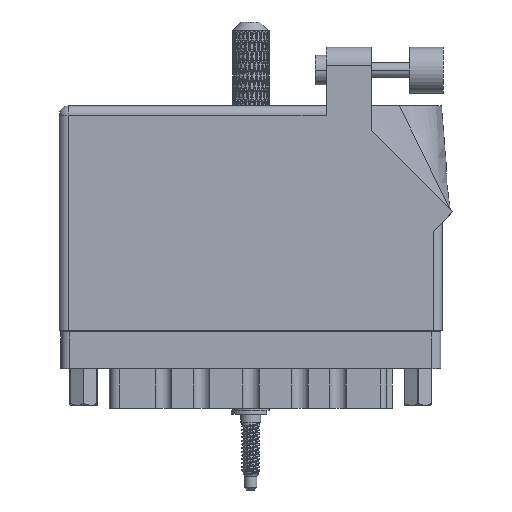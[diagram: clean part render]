
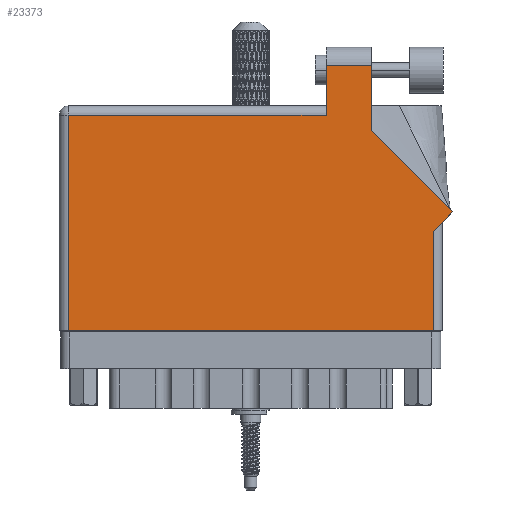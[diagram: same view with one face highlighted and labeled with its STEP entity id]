
A CAD part, front view. The second image highlights one B-rep face of the part: STEP entity #23373.
In plain terms, the highlighted face is planar.
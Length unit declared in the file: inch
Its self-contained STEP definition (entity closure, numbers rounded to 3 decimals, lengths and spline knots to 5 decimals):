
#1160 = DIRECTION ( 'NONE',  ( 0., 0., -1. ) ) ;
#1445 = VERTEX_POINT ( 'NONE', #15728 ) ;
#2718 = CARTESIAN_POINT ( 'NONE',  ( 0.062, 0., 0. ) ) ;
#2809 = CARTESIAN_POINT ( 'NONE',  ( 2.55, 0., 0. ) ) ;
#8725 = EDGE_CURVE ( 'NONE', #46012, #100111, #115693, .T. ) ;
#9694 = DIRECTION ( 'NONE',  ( 1., 0., 0. ) ) ;
#10680 = DIRECTION ( 'NONE',  ( -1., 0., 0. ) ) ;
#15728 = CARTESIAN_POINT ( 'NONE',  ( 2.55, 0.675, 0. ) ) ;
#22174 = LINE ( 'NONE', #75197, #93728 ) ;
#22695 = DIRECTION ( 'NONE',  ( 0., 1., 0. ) ) ;
#23373 = ADVANCED_FACE ( 'NONE', ( #100048 ), #78764, .F. ) ;
#23724 = VECTOR ( 'NONE', #22695, 39.37008 ) ;
#24155 = EDGE_CURVE ( 'NONE', #119926, #46796, #34147, .T. ) ;
#25047 = LINE ( 'NONE', #74549, #72838 ) ;
#26389 = LINE ( 'NONE', #67355, #39876 ) ;
#30416 = CARTESIAN_POINT ( 'NONE',  ( 0., 1.468, 0. ) ) ;
#32674 = CARTESIAN_POINT ( 'NONE',  ( 2.68271, 0.80771, 0. ) ) ;
#34147 = LINE ( 'NONE', #80301, #23724 ) ;
#36183 = DIRECTION ( 'NONE',  ( 0.707, 0.707, 0. ) ) ;
#39404 = CARTESIAN_POINT ( 'NONE',  ( 0., 0., 0. ) ) ;
#39876 = VECTOR ( 'NONE', #46555, 39.37008 ) ;
#40272 = DIRECTION ( 'NONE',  ( -0.707, 0.707, 0. ) ) ;
#43298 = ORIENTED_EDGE ( 'NONE', *, *, #79503, .T. ) ;
#46012 = VERTEX_POINT ( 'NONE', #2718 ) ;
#46555 = DIRECTION ( 'NONE',  ( 0., -1., 0. ) ) ;
#46796 = VERTEX_POINT ( 'NONE', #100819 ) ;
#49340 = EDGE_CURVE ( 'NONE', #68187, #119926, #106894, .T. ) ;
#50073 = ORIENTED_EDGE ( 'NONE', *, *, #8725, .T. ) ;
#50789 = CARTESIAN_POINT ( 'NONE',  ( 0., 1.53, 0. ) ) ;
#54359 = VERTEX_POINT ( 'NONE', #75942 ) ;
#60581 = CARTESIAN_POINT ( 'NONE',  ( 2.55, 0.737, 0. ) ) ;
#61415 = VECTOR ( 'NONE', #120790, 39.37008 ) ;
#67150 = DIRECTION ( 'NONE',  ( -1., 0., 0. ) ) ;
#67355 = CARTESIAN_POINT ( 'NONE',  ( 0.062, 0., 0. ) ) ;
#68187 = VERTEX_POINT ( 'NONE', #120037 ) ;
#69069 = EDGE_CURVE ( 'NONE', #54359, #46012, #26389, .T. ) ;
#70728 = ORIENTED_EDGE ( 'NONE', *, *, #115049, .T. ) ;
#72074 = CARTESIAN_POINT ( 'NONE',  ( 1.819, 1.805, 0. ) ) ;
#72685 = CARTESIAN_POINT ( 'NONE',  ( 1.819, 1.468, 0. ) ) ;
#72838 = VECTOR ( 'NONE', #36183, 39.37008 ) ;
#74119 = EDGE_CURVE ( 'NONE', #46796, #106268, #95720, .T. ) ;
#74367 = ORIENTED_EDGE ( 'NONE', *, *, #49340, .T. ) ;
#74549 = CARTESIAN_POINT ( 'NONE',  ( 2.612, 0.737, 0. ) ) ;
#75197 = CARTESIAN_POINT ( 'NONE',  ( 1.819, 1.53, 0. ) ) ;
#75942 = CARTESIAN_POINT ( 'NONE',  ( 0.062, 1.468, 0. ) ) ;
#76597 = ORIENTED_EDGE ( 'NONE', *, *, #69069, .T. ) ;
#78764 = PLANE ( 'NONE',  #100450 ) ;
#79074 = ORIENTED_EDGE ( 'NONE', *, *, #114481, .T. ) ;
#79503 = EDGE_CURVE ( 'NONE', #100111, #1445, #104712, .T. ) ;
#80206 = DIRECTION ( 'NONE',  ( 0., 1., 0. ) ) ;
#80301 = CARTESIAN_POINT ( 'NONE',  ( 2.126, 1.36442, 0. ) ) ;
#83221 = VECTOR ( 'NONE', #67150, 39.37008 ) ;
#90413 = VECTOR ( 'NONE', #9694, 39.37008 ) ;
#90846 = EDGE_CURVE ( 'NONE', #111351, #54359, #118954, .T. ) ;
#91414 = VECTOR ( 'NONE', #80206, 39.37008 ) ;
#93728 = VECTOR ( 'NONE', #105547, 39.37008 ) ;
#95720 = LINE ( 'NONE', #72074, #61415 ) ;
#100048 = FACE_OUTER_BOUND ( 'NONE', #108506, .T. ) ;
#100111 = VERTEX_POINT ( 'NONE', #2809 ) ;
#100450 = AXIS2_PLACEMENT_3D ( 'NONE', #50789, #1160, #10680 ) ;
#100819 = CARTESIAN_POINT ( 'NONE',  ( 2.126, 1.805, 0. ) ) ;
#104712 = LINE ( 'NONE', #60581, #91414 ) ;
#105547 = DIRECTION ( 'NONE',  ( 0., -1., 0. ) ) ;
#106268 = VERTEX_POINT ( 'NONE', #114165 ) ;
#106894 = LINE ( 'NONE', #32674, #111502 ) ;
#107000 = ORIENTED_EDGE ( 'NONE', *, *, #90846, .T. ) ;
#108506 = EDGE_LOOP ( 'NONE', ( #117914, #122545, #79074, #107000, #76597, #50073, #43298, #70728, #74367 ) ) ;
#110491 = CARTESIAN_POINT ( 'NONE',  ( 2.126, 1.36442, 0. ) ) ;
#111351 = VERTEX_POINT ( 'NONE', #72685 ) ;
#111502 = VECTOR ( 'NONE', #40272, 39.37008 ) ;
#114165 = CARTESIAN_POINT ( 'NONE',  ( 1.819, 1.805, 0. ) ) ;
#114481 = EDGE_CURVE ( 'NONE', #106268, #111351, #22174, .T. ) ;
#115049 = EDGE_CURVE ( 'NONE', #1445, #68187, #25047, .T. ) ;
#115693 = LINE ( 'NONE', #39404, #90413 ) ;
#117914 = ORIENTED_EDGE ( 'NONE', *, *, #24155, .T. ) ;
#118954 = LINE ( 'NONE', #30416, #83221 ) ;
#119926 = VERTEX_POINT ( 'NONE', #110491 ) ;
#120037 = CARTESIAN_POINT ( 'NONE',  ( 2.68271, 0.80771, 0. ) ) ;
#120790 = DIRECTION ( 'NONE',  ( -1., 0., 0. ) ) ;
#122545 = ORIENTED_EDGE ( 'NONE', *, *, #74119, .T. ) ;
